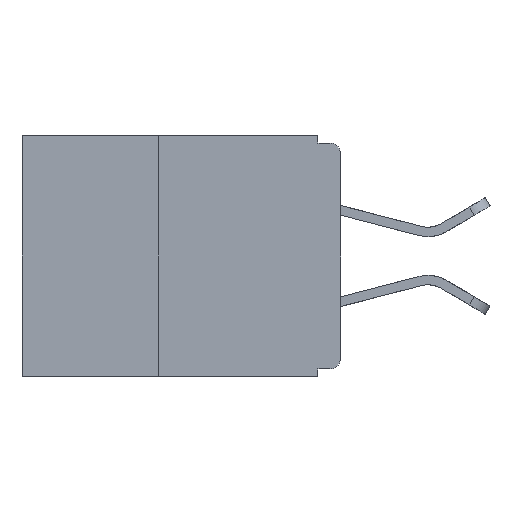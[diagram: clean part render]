
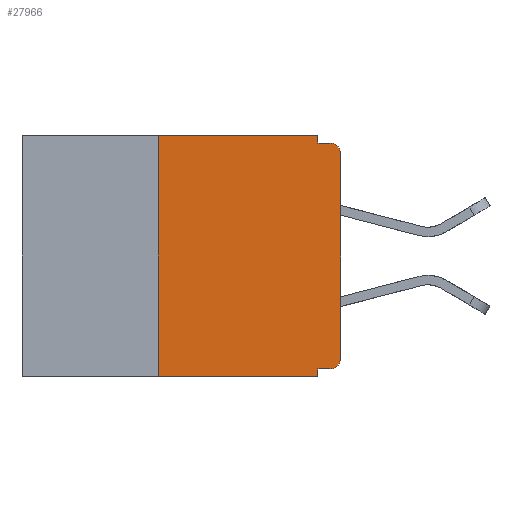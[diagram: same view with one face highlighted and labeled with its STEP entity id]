
A CAD part, left-side view. The second image highlights one B-rep face of the part: STEP entity #27966.
In plain terms, the highlighted planar face has unit normal (-1, 0, 0).
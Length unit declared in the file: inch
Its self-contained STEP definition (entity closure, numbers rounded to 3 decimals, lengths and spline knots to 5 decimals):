
#140 = ORIENTED_EDGE ( 'NONE', *, *, #6539, .F. ) ;
#461 = CARTESIAN_POINT ( 'NONE',  ( 0., 0., -0.305 ) ) ;
#540 = ORIENTED_EDGE ( 'NONE', *, *, #17226, .F. ) ;
#1055 = ORIENTED_EDGE ( 'NONE', *, *, #11089, .F. ) ;
#1593 = CARTESIAN_POINT ( 'NONE',  ( 0., 0.015, -0.01 ) ) ;
#1945 = CARTESIAN_POINT ( 'NONE',  ( 0., 0.031, 0. ) ) ;
#2217 = CARTESIAN_POINT ( 'NONE',  ( 0., 0.25, 0. ) ) ;
#2772 = ORIENTED_EDGE ( 'NONE', *, *, #27023, .F. ) ;
#2953 = ORIENTED_EDGE ( 'NONE', *, *, #24600, .T. ) ;
#3368 = VECTOR ( 'NONE', #9549, 39.37008 ) ;
#4214 = CARTESIAN_POINT ( 'NONE',  ( 0., 0.25, -0.33 ) ) ;
#4312 = DIRECTION ( 'NONE',  ( 0., 0., -1. ) ) ;
#4997 = VERTEX_POINT ( 'NONE', #19283 ) ;
#5543 = ORIENTED_EDGE ( 'NONE', *, *, #6471, .T. ) ;
#5900 = VECTOR ( 'NONE', #18110, 39.37008 ) ;
#6471 = EDGE_CURVE ( 'NONE', #14321, #4997, #12426, .T. ) ;
#6539 = EDGE_CURVE ( 'NONE', #6793, #21945, #10257, .T. ) ;
#6793 = VERTEX_POINT ( 'NONE', #23300 ) ;
#7082 = EDGE_CURVE ( 'NONE', #23178, #21945, #19521, .T. ) ;
#7483 = ORIENTED_EDGE ( 'NONE', *, *, #23994, .F. ) ;
#7791 = VERTEX_POINT ( 'NONE', #2217 ) ;
#8277 = AXIS2_PLACEMENT_3D ( 'NONE', #12657, #28682, #14968 ) ;
#8983 = AXIS2_PLACEMENT_3D ( 'NONE', #12312, #28347, #14610 ) ;
#8999 = CARTESIAN_POINT ( 'NONE',  ( 0., 0., -0.025 ) ) ;
#9125 = DIRECTION ( 'NONE',  ( -1., 0., 0. ) ) ;
#9549 = DIRECTION ( 'NONE',  ( 0., 1., 0. ) ) ;
#9861 = CARTESIAN_POINT ( 'NONE',  ( 0., 0.031, -0.32 ) ) ;
#10257 = LINE ( 'NONE', #15624, #22423 ) ;
#10932 = LINE ( 'NONE', #1945, #28489 ) ;
#11034 = LINE ( 'NONE', #25601, #3368 ) ;
#11089 = EDGE_CURVE ( 'NONE', #14321, #7791, #24219, .T. ) ;
#12312 = CARTESIAN_POINT ( 'NONE',  ( 0., 0.015, -0.305 ) ) ;
#12426 = LINE ( 'NONE', #19911, #17778 ) ;
#12656 = VECTOR ( 'NONE', #24302, 39.37008 ) ;
#12657 = CARTESIAN_POINT ( 'NONE',  ( 0., 0.437, 0. ) ) ;
#12822 = CARTESIAN_POINT ( 'NONE',  ( 0., 0.015, -0.32 ) ) ;
#12867 = CARTESIAN_POINT ( 'NONE',  ( 0., 0., 0. ) ) ;
#13077 = EDGE_CURVE ( 'NONE', #25224, #23178, #18021, .T. ) ;
#13105 = DIRECTION ( 'NONE',  ( 0., -1., 0. ) ) ;
#13397 = LINE ( 'NONE', #23802, #17328 ) ;
#14321 = VERTEX_POINT ( 'NONE', #24011 ) ;
#14610 = DIRECTION ( 'NONE',  ( 0., 0., -1. ) ) ;
#14968 = DIRECTION ( 'NONE',  ( 0., 0., -1. ) ) ;
#15138 = EDGE_LOOP ( 'NONE', ( #17545, #23161, #140, #540, #24409, #1055, #5543, #2772, #7483, #2953 ) ) ;
#15240 = VECTOR ( 'NONE', #15586, 39.37008 ) ;
#15586 = DIRECTION ( 'NONE',  ( 0., -1., 0. ) ) ;
#15624 = CARTESIAN_POINT ( 'NONE',  ( 0., 0., -0.01 ) ) ;
#16890 = DIRECTION ( 'NONE',  ( 0., 0., -1. ) ) ;
#17226 = EDGE_CURVE ( 'NONE', #22481, #6793, #10932, .T. ) ;
#17328 = VECTOR ( 'NONE', #16890, 39.37008 ) ;
#17545 = ORIENTED_EDGE ( 'NONE', *, *, #13077, .T. ) ;
#17546 = CARTESIAN_POINT ( 'NONE',  ( 0., 0.031, 0. ) ) ;
#17778 = VECTOR ( 'NONE', #13105, 39.37008 ) ;
#18021 = LINE ( 'NONE', #12867, #12656 ) ;
#18110 = DIRECTION ( 'NONE',  ( 0., 0., 1. ) ) ;
#19283 = CARTESIAN_POINT ( 'NONE',  ( 0., 0.031, -0.33 ) ) ;
#19521 = CIRCLE ( 'NONE', #26055, 0.015 ) ;
#19911 = CARTESIAN_POINT ( 'NONE',  ( 0., 0.437, -0.33 ) ) ;
#20128 = VERTEX_POINT ( 'NONE', #9861 ) ;
#21298 = LINE ( 'NONE', #29271, #15240 ) ;
#21750 = PLANE ( 'NONE',  #8277 ) ;
#21945 = VERTEX_POINT ( 'NONE', #1593 ) ;
#22423 = VECTOR ( 'NONE', #29305, 39.37008 ) ;
#22481 = VERTEX_POINT ( 'NONE', #17546 ) ;
#22829 = CARTESIAN_POINT ( 'NONE',  ( 0., 0.015, -0.025 ) ) ;
#23161 = ORIENTED_EDGE ( 'NONE', *, *, #7082, .T. ) ;
#23178 = VERTEX_POINT ( 'NONE', #8999 ) ;
#23300 = CARTESIAN_POINT ( 'NONE',  ( 0., 0.031, -0.01 ) ) ;
#23802 = CARTESIAN_POINT ( 'NONE',  ( 0., 0.031, -0.33 ) ) ;
#23994 = EDGE_CURVE ( 'NONE', #28632, #20128, #11034, .T. ) ;
#24011 = CARTESIAN_POINT ( 'NONE',  ( 0., 0.25, -0.33 ) ) ;
#24219 = LINE ( 'NONE', #4214, #5900 ) ;
#24302 = DIRECTION ( 'NONE',  ( 0., 0., 1. ) ) ;
#24409 = ORIENTED_EDGE ( 'NONE', *, *, #25538, .F. ) ;
#24600 = EDGE_CURVE ( 'NONE', #28632, #25224, #25704, .T. ) ;
#25183 = DIRECTION ( 'NONE',  ( 0., 0., -1. ) ) ;
#25224 = VERTEX_POINT ( 'NONE', #461 ) ;
#25538 = EDGE_CURVE ( 'NONE', #7791, #22481, #21298, .T. ) ;
#25601 = CARTESIAN_POINT ( 'NONE',  ( 0., 0., -0.32 ) ) ;
#25704 = CIRCLE ( 'NONE', #8983, 0.015 ) ;
#26055 = AXIS2_PLACEMENT_3D ( 'NONE', #22829, #9125, #25183 ) ;
#27023 = EDGE_CURVE ( 'NONE', #20128, #4997, #13397, .T. ) ;
#27966 = ADVANCED_FACE ( 'NONE', ( #28731 ), #21750, .F. ) ;
#28347 = DIRECTION ( 'NONE',  ( -1., 0., 0. ) ) ;
#28489 = VECTOR ( 'NONE', #4312, 39.37008 ) ;
#28632 = VERTEX_POINT ( 'NONE', #12822 ) ;
#28682 = DIRECTION ( 'NONE',  ( 1., 0., 0. ) ) ;
#28731 = FACE_OUTER_BOUND ( 'NONE', #15138, .T. ) ;
#29271 = CARTESIAN_POINT ( 'NONE',  ( 0., 0.437, 0. ) ) ;
#29305 = DIRECTION ( 'NONE',  ( 0., -1., 0. ) ) ;
